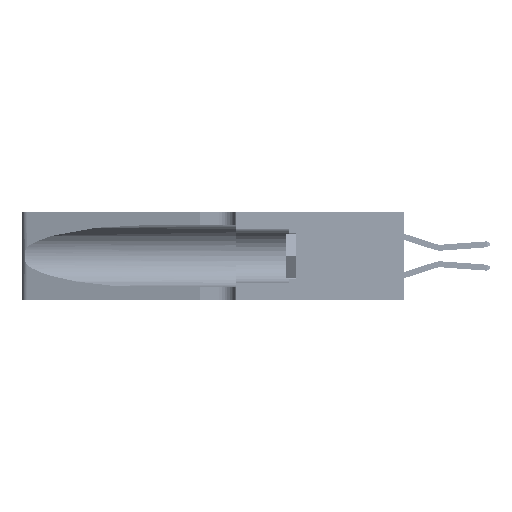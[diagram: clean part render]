
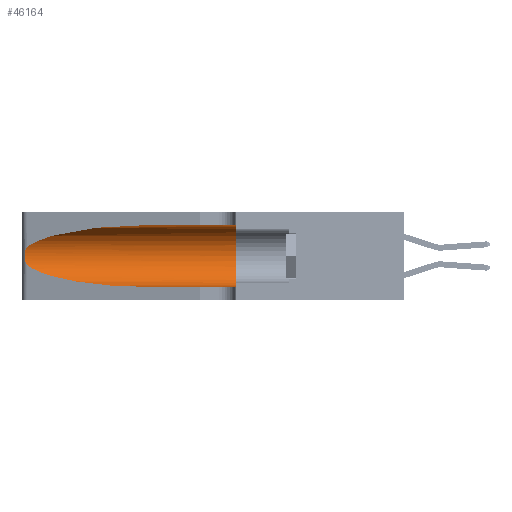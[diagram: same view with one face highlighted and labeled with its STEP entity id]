
A CAD part, left-side view. The second image highlights one B-rep face of the part: STEP entity #46164.
In plain terms, the highlighted cylindrical face has radius 3.308 mm (diameter 6.617 mm), a partial arc.
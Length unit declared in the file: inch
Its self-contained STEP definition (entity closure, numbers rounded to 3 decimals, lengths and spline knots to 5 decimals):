
#833 = CARTESIAN_POINT ( 'NONE',  ( 0.25639, 1.23184, 0.21858 ) ) ;
#863 =( BOUNDED_CURVE ( )  B_SPLINE_CURVE ( 3, ( #40835, #37477, #30029, #37149 ),
 .UNSPECIFIED., .F., .T. ) 
 B_SPLINE_CURVE_WITH_KNOTS ( ( 4, 4 ),
 ( 3.44316, 4.71239 ),
 .UNSPECIFIED. ) 
 CURVE ( )  GEOMETRIC_REPRESENTATION_ITEM ( )  RATIONAL_B_SPLINE_CURVE ( ( 1., 0.87, 0.87, 1. ) ) 
 REPRESENTATION_ITEM ( '' )  );
#1019 = CARTESIAN_POINT ( 'NONE',  ( 0.1305, 0.72297, 0.31525 ) ) ;
#1218 = ORIENTED_EDGE ( 'NONE', *, *, #30824, .T. ) ;
#3166 = DIRECTION ( 'NONE',  ( 0., 0., -1. ) ) ;
#3321 = CARTESIAN_POINT ( 'NONE',  ( 0.2373, 1.15595, 0.28018 ) ) ;
#4081 = VERTEX_POINT ( 'NONE', #12419 ) ;
#4803 = CARTESIAN_POINT ( 'NONE',  ( 0.26018, 1.23835, 0.19895 ) ) ;
#5291 = CARTESIAN_POINT ( 'NONE',  ( 0.25856, 1.23593, 0.16098 ) ) ;
#5444 = CARTESIAN_POINT ( 'NONE',  ( 0.26017, 1.23833, 0.17102 ) ) ;
#5889 = DIRECTION ( 'NONE',  ( 0., -1., 0. ) ) ;
#6014 = CARTESIAN_POINT ( 'NONE',  ( 0.1305, 1.61858, 0.05475 ) ) ;
#6110 = EDGE_LOOP ( 'NONE', ( #1218, #11640, #40830, #38364, #21770, #19793 ) ) ;
#6368 = DIRECTION ( 'NONE',  ( 0., -1., 0. ) ) ;
#7464 = LINE ( 'NONE', #6014, #13348 ) ;
#8602 = CARTESIAN_POINT ( 'NONE',  ( 0.26075, 1.23896, 0.19203 ) ) ;
#9948 = DIRECTION ( 'NONE',  ( 0., -1., 0. ) ) ;
#10350 = LINE ( 'NONE', #48163, #42912 ) ;
#11640 = ORIENTED_EDGE ( 'NONE', *, *, #36970, .T. ) ;
#12419 = CARTESIAN_POINT ( 'NONE',  ( 0.25487, 1.22718, 0.14631 ) ) ;
#13348 = VECTOR ( 'NONE', #5889, 39.37008 ) ;
#13768 = CARTESIAN_POINT ( 'NONE',  ( 0.1305, 0.35, 0.05475 ) ) ;
#14467 = EDGE_CURVE ( 'NONE', #42075, #40942, #7464, .T. ) ;
#16274 = DIRECTION ( 'NONE',  ( 0., 1., 0. ) ) ;
#16318 = CARTESIAN_POINT ( 'NONE',  ( 0.25555, 1.22993, 0.14849 ) ) ;
#16452 = DIRECTION ( 'NONE',  ( 0., 0., 1. ) ) ;
#16800 = EDGE_CURVE ( 'NONE', #4081, #42075, #863, .T. ) ;
#18721 = CIRCLE ( 'NONE', #22365, 0.13025 ) ;
#19793 = ORIENTED_EDGE ( 'NONE', *, *, #44819, .F. ) ;
#21430 =( BOUNDED_CURVE ( )  B_SPLINE_CURVE ( 3, ( #25792, #34053, #3321, #26117 ),
 .UNSPECIFIED., .F., .T. ) 
 B_SPLINE_CURVE_WITH_KNOTS ( ( 4, 4 ),
 ( 1.5708, 2.84003 ),
 .UNSPECIFIED. ) 
 CURVE ( )  GEOMETRIC_REPRESENTATION_ITEM ( )  RATIONAL_B_SPLINE_CURVE ( ( 1., 0.87, 0.87, 1. ) ) 
 REPRESENTATION_ITEM ( '' )  );
#21770 = ORIENTED_EDGE ( 'NONE', *, *, #42676, .F. ) ;
#22365 = AXIS2_PLACEMENT_3D ( 'NONE', #35158, #16274, #16452 ) ;
#22717 = VERTEX_POINT ( 'NONE', #1019 ) ;
#25792 = CARTESIAN_POINT ( 'NONE',  ( 0.1305, 0.72297, 0.31525 ) ) ;
#26117 = CARTESIAN_POINT ( 'NONE',  ( 0.25487, 1.22718, 0.22369 ) ) ;
#26589 = AXIS2_PLACEMENT_3D ( 'NONE', #46950, #6368, #3166 ) ;
#26727 = CYLINDRICAL_SURFACE ( 'NONE', #26589, 0.13025 ) ;
#27443 = CARTESIAN_POINT ( 'NONE',  ( 0.25854, 1.2359, 0.20912 ) ) ;
#27914 = FACE_OUTER_BOUND ( 'NONE', #6110, .T. ) ;
#30029 = CARTESIAN_POINT ( 'NONE',  ( 0.18966, 0.96281, 0.05475 ) ) ;
#30824 = EDGE_CURVE ( 'NONE', #22717, #36550, #21430, .T. ) ;
#32057 = CARTESIAN_POINT ( 'NONE',  ( 0.25639, 1.23186, 0.15144 ) ) ;
#32597 = CARTESIAN_POINT ( 'NONE',  ( 0.1305, 0.35, 0.31525 ) ) ;
#34053 = CARTESIAN_POINT ( 'NONE',  ( 0.18966, 0.96281, 0.31525 ) ) ;
#34713 = CARTESIAN_POINT ( 'NONE',  ( 0.25487, 1.22718, 0.22369 ) ) ;
#35158 = CARTESIAN_POINT ( 'NONE',  ( 0.1305, 0.35, 0.185 ) ) ;
#36550 = VERTEX_POINT ( 'NONE', #40511 ) ;
#36970 = EDGE_CURVE ( 'NONE', #36550, #4081, #40594, .T. ) ;
#37149 = CARTESIAN_POINT ( 'NONE',  ( 0.1305, 0.72297, 0.05475 ) ) ;
#37477 = CARTESIAN_POINT ( 'NONE',  ( 0.2373, 1.15595, 0.08982 ) ) ;
#38364 = ORIENTED_EDGE ( 'NONE', *, *, #14467, .T. ) ;
#39360 = CARTESIAN_POINT ( 'NONE',  ( 0.25789, 1.23486, 0.15765 ) ) ;
#40511 = CARTESIAN_POINT ( 'NONE',  ( 0.25487, 1.22718, 0.22369 ) ) ;
#40594 = B_SPLINE_CURVE_WITH_KNOTS ( 'NONE', 3,
 ( #34713, #42525, #833, #46333, #27443, #4803, #8602, #46654, #5444, #5291, #39360, #32057, #16318, #47139 ),
 .UNSPECIFIED., .F., .F.,
 ( 4, 2, 2, 2, 2, 2, 4 ),
 ( 0., 0.00027, 0.00053, 0.00107, 0.0016, 0.00187, 0.00214 ),
 .UNSPECIFIED. ) ;
#40830 = ORIENTED_EDGE ( 'NONE', *, *, #16800, .T. ) ;
#40835 = CARTESIAN_POINT ( 'NONE',  ( 0.25487, 1.22718, 0.14631 ) ) ;
#40942 = VERTEX_POINT ( 'NONE', #13768 ) ;
#42075 = VERTEX_POINT ( 'NONE', #47648 ) ;
#42525 = CARTESIAN_POINT ( 'NONE',  ( 0.25555, 1.22994, 0.2215 ) ) ;
#42676 = EDGE_CURVE ( 'NONE', #47029, #40942, #18721, .T. ) ;
#42912 = VECTOR ( 'NONE', #9948, 39.37008 ) ;
#44819 = EDGE_CURVE ( 'NONE', #22717, #47029, #10350, .T. ) ;
#46164 = ADVANCED_FACE ( 'NONE', ( #27914 ), #26727, .F. ) ;
#46333 = CARTESIAN_POINT ( 'NONE',  ( 0.25787, 1.23484, 0.2124 ) ) ;
#46654 = CARTESIAN_POINT ( 'NONE',  ( 0.26075, 1.23896, 0.178 ) ) ;
#46950 = CARTESIAN_POINT ( 'NONE',  ( 0.1305, 1.61858, 0.185 ) ) ;
#47029 = VERTEX_POINT ( 'NONE', #32597 ) ;
#47139 = CARTESIAN_POINT ( 'NONE',  ( 0.25487, 1.22718, 0.14631 ) ) ;
#47648 = CARTESIAN_POINT ( 'NONE',  ( 0.1305, 0.72297, 0.05475 ) ) ;
#48163 = CARTESIAN_POINT ( 'NONE',  ( 0.1305, 1.61858, 0.31525 ) ) ;
